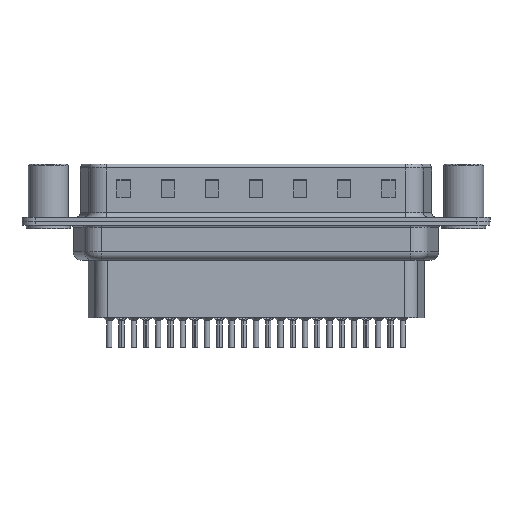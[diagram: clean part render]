
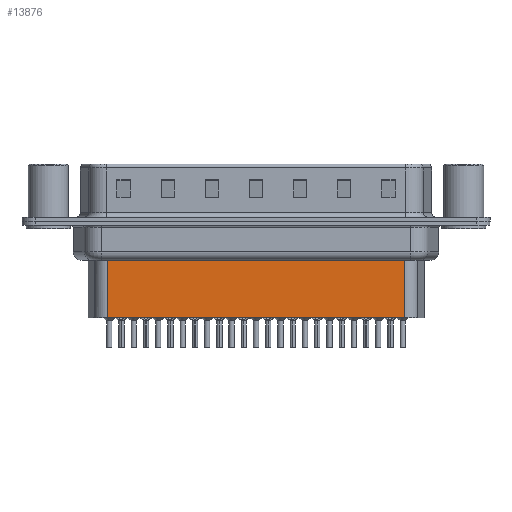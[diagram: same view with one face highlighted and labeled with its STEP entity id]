
A CAD part, front view. The second image highlights one B-rep face of the part: STEP entity #13876.
In plain terms, the highlighted planar face has unit normal (0, -1, 0).
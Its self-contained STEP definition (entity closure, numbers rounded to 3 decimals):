
#43 = CARTESIAN_POINT ( 'NONE',  ( 6.706, -3.5, -4.097 ) ) ;
#766 = CARTESIAN_POINT ( 'NONE',  ( 6.706, -3.5, -3.1 ) ) ;
#1039 = VECTOR ( 'NONE', #23409, 1000. ) ;
#1655 = CARTESIAN_POINT ( 'NONE',  ( 40.344, -3.5, -4.097 ) ) ;
#2020 = ORIENTED_EDGE ( 'NONE', *, *, #24724, .F. ) ;
#2035 = LINE ( 'NONE', #5707, #10057 ) ;
#3071 = EDGE_CURVE ( 'NONE', #20913, #11266, #9906, .T. ) ;
#4407 = AXIS2_PLACEMENT_3D ( 'NONE', #766, #22675, #4689 ) ;
#4689 = DIRECTION ( 'NONE',  ( 1., 0., 0. ) ) ;
#5519 = CARTESIAN_POINT ( 'NONE',  ( 40.344, -3.5, -3.1 ) ) ;
#5707 = CARTESIAN_POINT ( 'NONE',  ( 6.459, -3.5, -4.097 ) ) ;
#5910 = VERTEX_POINT ( 'NONE', #7095 ) ;
#6150 = VECTOR ( 'NONE', #17715, 1000. ) ;
#7095 = CARTESIAN_POINT ( 'NONE',  ( 40.344, -3.5, -10.95 ) ) ;
#7303 = CARTESIAN_POINT ( 'NONE',  ( 6.706, -3.5, -10.95 ) ) ;
#9906 = LINE ( 'NONE', #17909, #23153 ) ;
#10039 = DIRECTION ( 'NONE',  ( 0., 0., -1. ) ) ;
#10048 = VERTEX_POINT ( 'NONE', #1655 ) ;
#10057 = VECTOR ( 'NONE', #21737, 1000. ) ;
#11266 = VERTEX_POINT ( 'NONE', #7303 ) ;
#12207 = EDGE_CURVE ( 'NONE', #10048, #5910, #17449, .T. ) ;
#13283 = LINE ( 'NONE', #21574, #1039 ) ;
#13876 = ADVANCED_FACE ( 'NONE', ( #14771 ), #18729, .T. ) ;
#14771 = FACE_OUTER_BOUND ( 'NONE', #22035, .T. ) ;
#17126 = ORIENTED_EDGE ( 'NONE', *, *, #18770, .T. ) ;
#17449 = LINE ( 'NONE', #5519, #6150 ) ;
#17715 = DIRECTION ( 'NONE',  ( 0., 0., -1. ) ) ;
#17909 = CARTESIAN_POINT ( 'NONE',  ( 6.706, -3.5, -3.1 ) ) ;
#18729 = PLANE ( 'NONE',  #4407 ) ;
#18770 = EDGE_CURVE ( 'NONE', #10048, #20913, #2035, .T. ) ;
#20532 = ORIENTED_EDGE ( 'NONE', *, *, #12207, .F. ) ;
#20913 = VERTEX_POINT ( 'NONE', #43 ) ;
#21574 = CARTESIAN_POINT ( 'NONE',  ( 6.706, -3.5, -10.95 ) ) ;
#21737 = DIRECTION ( 'NONE',  ( -1., 0., 0. ) ) ;
#22035 = EDGE_LOOP ( 'NONE', ( #20532, #17126, #24743, #2020 ) ) ;
#22675 = DIRECTION ( 'NONE',  ( 0., -1., 0. ) ) ;
#23153 = VECTOR ( 'NONE', #10039, 1000. ) ;
#23409 = DIRECTION ( 'NONE',  ( -1., 0., 0. ) ) ;
#24724 = EDGE_CURVE ( 'NONE', #5910, #11266, #13283, .T. ) ;
#24743 = ORIENTED_EDGE ( 'NONE', *, *, #3071, .T. ) ;
